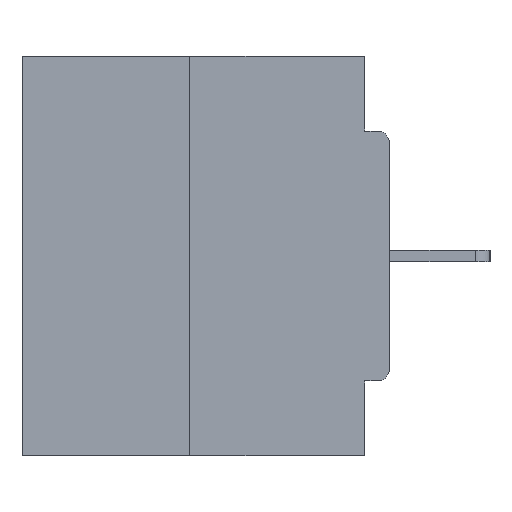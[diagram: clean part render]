
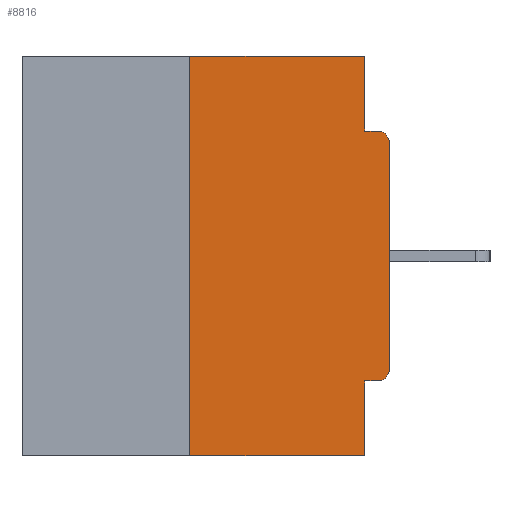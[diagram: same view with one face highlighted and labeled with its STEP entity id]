
A CAD part, left-side view. The second image highlights one B-rep face of the part: STEP entity #8816.
In plain terms, the highlighted planar face has unit normal (-1, 0, 0).
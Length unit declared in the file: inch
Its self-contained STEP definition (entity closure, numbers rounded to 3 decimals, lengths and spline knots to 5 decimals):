
#145 = VERTEX_POINT ( 'NONE', #13634 ) ;
#352 = ORIENTED_EDGE ( 'NONE', *, *, #19380, .T. ) ;
#416 = DIRECTION ( 'NONE',  ( -1., 0., 0. ) ) ;
#420 = ORIENTED_EDGE ( 'NONE', *, *, #27150, .F. ) ;
#683 = EDGE_CURVE ( 'NONE', #5086, #17890, #9795, .T. ) ;
#790 = CARTESIAN_POINT ( 'NONE',  ( 0., 0.46, 0. ) ) ;
#1380 = DIRECTION ( 'NONE',  ( 0., 0., -1. ) ) ;
#1421 = VERTEX_POINT ( 'NONE', #13483 ) ;
#1527 = VERTEX_POINT ( 'NONE', #9535 ) ;
#2561 = CARTESIAN_POINT ( 'NONE',  ( 0., 0.25, 0. ) ) ;
#2753 = CARTESIAN_POINT ( 'NONE',  ( 0., 0.46, 0. ) ) ;
#3007 = CARTESIAN_POINT ( 'NONE',  ( 0., 0.46, -0.5 ) ) ;
#3164 = EDGE_CURVE ( 'NONE', #145, #1421, #27824, .T. ) ;
#3383 = LINE ( 'NONE', #17722, #20693 ) ;
#3840 = LINE ( 'NONE', #12534, #7556 ) ;
#4020 = DIRECTION ( 'NONE',  ( 0., 1., 0. ) ) ;
#4233 = CARTESIAN_POINT ( 'NONE',  ( 0., 0.031, -0.4065 ) ) ;
#5086 = VERTEX_POINT ( 'NONE', #2561 ) ;
#5239 = DIRECTION ( 'NONE',  ( 1., 0., 0. ) ) ;
#5337 = EDGE_CURVE ( 'NONE', #25246, #1421, #17967, .T. ) ;
#5357 = VERTEX_POINT ( 'NONE', #4233 ) ;
#5759 = DIRECTION ( 'NONE',  ( 0., -1., 0. ) ) ;
#6702 = EDGE_CURVE ( 'NONE', #20611, #10085, #23979, .T. ) ;
#7134 = DIRECTION ( 'NONE',  ( 0., 0., 1. ) ) ;
#7556 = VECTOR ( 'NONE', #1380, 39.37008 ) ;
#8262 = LINE ( 'NONE', #27103, #25878 ) ;
#8635 = VECTOR ( 'NONE', #4020, 39.37008 ) ;
#8681 = VECTOR ( 'NONE', #26189, 39.37008 ) ;
#8816 = ADVANCED_FACE ( 'NONE', ( #10570 ), #16829, .F. ) ;
#8956 = CARTESIAN_POINT ( 'NONE',  ( 0., 0.015, -0.4065 ) ) ;
#9535 = CARTESIAN_POINT ( 'NONE',  ( 0., 0., -0.3915 ) ) ;
#9795 = LINE ( 'NONE', #2753, #8681 ) ;
#10085 = VERTEX_POINT ( 'NONE', #22181 ) ;
#10352 = VERTEX_POINT ( 'NONE', #8956 ) ;
#10570 = FACE_OUTER_BOUND ( 'NONE', #23930, .T. ) ;
#11257 = ORIENTED_EDGE ( 'NONE', *, *, #683, .F. ) ;
#12260 = VECTOR ( 'NONE', #5759, 39.37008 ) ;
#12435 = EDGE_CURVE ( 'NONE', #17890, #25246, #3383, .T. ) ;
#12440 = ORIENTED_EDGE ( 'NONE', *, *, #6702, .T. ) ;
#12534 = CARTESIAN_POINT ( 'NONE',  ( 0., 0.031, -0.5 ) ) ;
#12543 = DIRECTION ( 'NONE',  ( 0., 0., -1. ) ) ;
#13483 = CARTESIAN_POINT ( 'NONE',  ( 0., 0.015, -0.0935 ) ) ;
#13634 = CARTESIAN_POINT ( 'NONE',  ( 0., 0., -0.1085 ) ) ;
#13663 = EDGE_CURVE ( 'NONE', #5357, #10085, #3840, .T. ) ;
#15661 = VECTOR ( 'NONE', #7134, 39.37008 ) ;
#16435 = EDGE_CURVE ( 'NONE', #10352, #5357, #22826, .T. ) ;
#16726 = ORIENTED_EDGE ( 'NONE', *, *, #16435, .F. ) ;
#16829 = PLANE ( 'NONE',  #18641 ) ;
#17194 = ORIENTED_EDGE ( 'NONE', *, *, #5337, .F. ) ;
#17722 = CARTESIAN_POINT ( 'NONE',  ( 0., 0.031, 0. ) ) ;
#17890 = VERTEX_POINT ( 'NONE', #23897 ) ;
#17967 = LINE ( 'NONE', #29815, #21673 ) ;
#18527 = CARTESIAN_POINT ( 'NONE',  ( 0., 0.015, -0.1085 ) ) ;
#18641 = AXIS2_PLACEMENT_3D ( 'NONE', #790, #5239, #12543 ) ;
#19380 = EDGE_CURVE ( 'NONE', #1527, #145, #8262, .T. ) ;
#19709 = EDGE_CURVE ( 'NONE', #10352, #1527, #24426, .T. ) ;
#19765 = CARTESIAN_POINT ( 'NONE',  ( 0., 0.25, -0.5 ) ) ;
#20179 = DIRECTION ( 'NONE',  ( 0., 0., 1. ) ) ;
#20518 = CARTESIAN_POINT ( 'NONE',  ( 0., 0., -0.4065 ) ) ;
#20586 = DIRECTION ( 'NONE',  ( 0., -1., 0. ) ) ;
#20611 = VERTEX_POINT ( 'NONE', #19765 ) ;
#20693 = VECTOR ( 'NONE', #28969, 39.37008 ) ;
#21353 = CARTESIAN_POINT ( 'NONE',  ( 0., 0.015, -0.3915 ) ) ;
#21673 = VECTOR ( 'NONE', #20586, 39.37008 ) ;
#22181 = CARTESIAN_POINT ( 'NONE',  ( 0., 0.031, -0.5 ) ) ;
#22826 = LINE ( 'NONE', #20518, #8635 ) ;
#23397 = AXIS2_PLACEMENT_3D ( 'NONE', #18527, #27924, #28371 ) ;
#23434 = AXIS2_PLACEMENT_3D ( 'NONE', #21353, #416, #26303 ) ;
#23897 = CARTESIAN_POINT ( 'NONE',  ( 0., 0.031, 0. ) ) ;
#23930 = EDGE_LOOP ( 'NONE', ( #11257, #420, #12440, #28012, #16726, #30074, #352, #25333, #17194, #26525 ) ) ;
#23979 = LINE ( 'NONE', #3007, #12260 ) ;
#24426 = CIRCLE ( 'NONE', #23434, 0.015 ) ;
#25246 = VERTEX_POINT ( 'NONE', #27045 ) ;
#25333 = ORIENTED_EDGE ( 'NONE', *, *, #3164, .T. ) ;
#25878 = VECTOR ( 'NONE', #20179, 39.37008 ) ;
#26189 = DIRECTION ( 'NONE',  ( 0., -1., 0. ) ) ;
#26303 = DIRECTION ( 'NONE',  ( 0., 0., -1. ) ) ;
#26386 = LINE ( 'NONE', #26530, #15661 ) ;
#26525 = ORIENTED_EDGE ( 'NONE', *, *, #12435, .F. ) ;
#26530 = CARTESIAN_POINT ( 'NONE',  ( 0., 0.25, 0. ) ) ;
#27045 = CARTESIAN_POINT ( 'NONE',  ( 0., 0.031, -0.0935 ) ) ;
#27103 = CARTESIAN_POINT ( 'NONE',  ( 0., 0., 0. ) ) ;
#27150 = EDGE_CURVE ( 'NONE', #20611, #5086, #26386, .T. ) ;
#27824 = CIRCLE ( 'NONE', #23397, 0.015 ) ;
#27924 = DIRECTION ( 'NONE',  ( -1., 0., 0. ) ) ;
#28012 = ORIENTED_EDGE ( 'NONE', *, *, #13663, .F. ) ;
#28371 = DIRECTION ( 'NONE',  ( 0., 0., -1. ) ) ;
#28969 = DIRECTION ( 'NONE',  ( 0., 0., -1. ) ) ;
#29815 = CARTESIAN_POINT ( 'NONE',  ( 0., 0., -0.0935 ) ) ;
#30074 = ORIENTED_EDGE ( 'NONE', *, *, #19709, .T. ) ;
